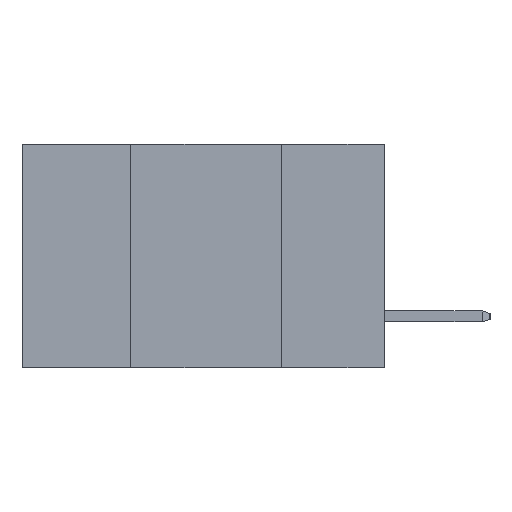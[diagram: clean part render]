
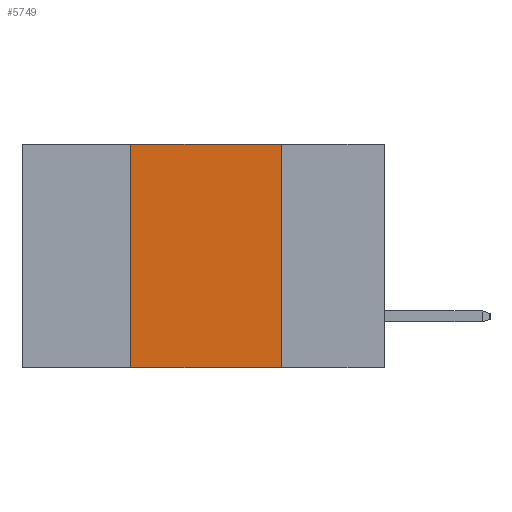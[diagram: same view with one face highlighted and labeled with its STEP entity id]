
A CAD part, left-side view. The second image highlights one B-rep face of the part: STEP entity #5749.
In plain terms, the highlighted planar face has unit normal (-1, 0, 0).
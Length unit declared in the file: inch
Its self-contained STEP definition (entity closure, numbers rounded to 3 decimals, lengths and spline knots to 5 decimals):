
#326 = DIRECTION ( 'NONE',  ( 1., 0., 0. ) ) ;
#343 = DIRECTION ( 'NONE',  ( 0., 0., -1. ) ) ;
#353 = EDGE_CURVE ( 'NONE', #10364, #8852, #2878, .T. ) ;
#393 = PLANE ( 'NONE',  #10874 ) ;
#901 = VECTOR ( 'NONE', #7910, 39.37008 ) ;
#945 = CARTESIAN_POINT ( 'NONE',  ( 0., 0.6, 0. ) ) ;
#1644 = CARTESIAN_POINT ( 'NONE',  ( 0., 0.17, -0.37 ) ) ;
#2106 = VECTOR ( 'NONE', #7054, 39.37008 ) ;
#2261 = VERTEX_POINT ( 'NONE', #10639 ) ;
#2274 = VECTOR ( 'NONE', #10557, 39.37008 ) ;
#2348 = CARTESIAN_POINT ( 'NONE',  ( 0., 0.42, -0.37 ) ) ;
#2366 = DIRECTION ( 'NONE',  ( 0., -1., 0. ) ) ;
#2878 = LINE ( 'NONE', #1644, #901 ) ;
#3313 = CARTESIAN_POINT ( 'NONE',  ( 0., 0.6, 0. ) ) ;
#4107 = VECTOR ( 'NONE', #2366, 39.37008 ) ;
#4146 = ORIENTED_EDGE ( 'NONE', *, *, #353, .F. ) ;
#5090 = LINE ( 'NONE', #2348, #2274 ) ;
#5449 = VERTEX_POINT ( 'NONE', #11268 ) ;
#5744 = ORIENTED_EDGE ( 'NONE', *, *, #10522, .T. ) ;
#5749 = ADVANCED_FACE ( 'NONE', ( #6589 ), #393, .F. ) ;
#5987 = CARTESIAN_POINT ( 'NONE',  ( 0., 0.17, -0.37 ) ) ;
#6093 = CARTESIAN_POINT ( 'NONE',  ( 0., 0.6, -0.37 ) ) ;
#6258 = LINE ( 'NONE', #6093, #4107 ) ;
#6589 = FACE_OUTER_BOUND ( 'NONE', #10600, .T. ) ;
#7054 = DIRECTION ( 'NONE',  ( 0., -1., 0. ) ) ;
#7110 = LINE ( 'NONE', #3313, #2106 ) ;
#7910 = DIRECTION ( 'NONE',  ( 0., 0., -1. ) ) ;
#8607 = CARTESIAN_POINT ( 'NONE',  ( 0., 0.17, 0. ) ) ;
#8852 = VERTEX_POINT ( 'NONE', #5987 ) ;
#8906 = ORIENTED_EDGE ( 'NONE', *, *, #11670, .F. ) ;
#10364 = VERTEX_POINT ( 'NONE', #8607 ) ;
#10372 = ORIENTED_EDGE ( 'NONE', *, *, #11100, .F. ) ;
#10522 = EDGE_CURVE ( 'NONE', #5449, #8852, #6258, .T. ) ;
#10557 = DIRECTION ( 'NONE',  ( 0., 0., 1. ) ) ;
#10600 = EDGE_LOOP ( 'NONE', ( #4146, #8906, #10372, #5744 ) ) ;
#10639 = CARTESIAN_POINT ( 'NONE',  ( 0., 0.42, 0. ) ) ;
#10874 = AXIS2_PLACEMENT_3D ( 'NONE', #945, #326, #343 ) ;
#11100 = EDGE_CURVE ( 'NONE', #5449, #2261, #5090, .T. ) ;
#11268 = CARTESIAN_POINT ( 'NONE',  ( 0., 0.42, -0.37 ) ) ;
#11670 = EDGE_CURVE ( 'NONE', #2261, #10364, #7110, .T. ) ;
